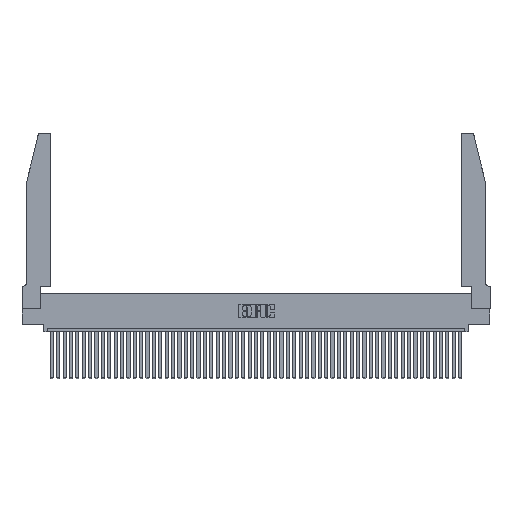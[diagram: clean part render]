
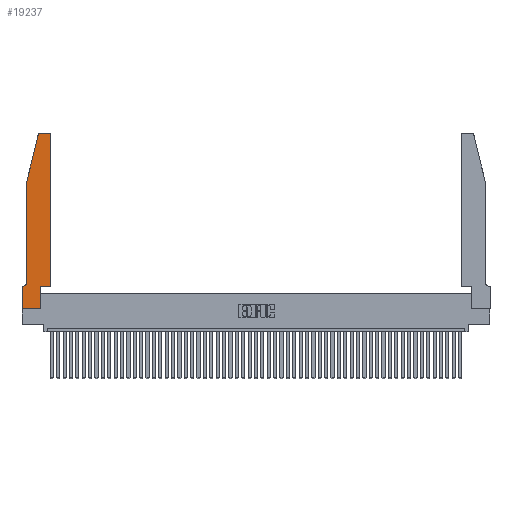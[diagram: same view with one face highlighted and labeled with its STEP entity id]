
A CAD part, top view. The second image highlights one B-rep face of the part: STEP entity #19237.
In plain terms, the highlighted planar face has unit normal (0, 0, 1).
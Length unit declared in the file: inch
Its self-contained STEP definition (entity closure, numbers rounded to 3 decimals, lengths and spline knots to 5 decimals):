
#61 = EDGE_CURVE ( 'NONE', #42414, #43759, #48741, .T. ) ;
#209 = ORIENTED_EDGE ( 'NONE', *, *, #61, .T. ) ;
#306 = CARTESIAN_POINT ( 'NONE',  ( 0.2865, 0.35, 0.37 ) ) ;
#961 = VERTEX_POINT ( 'NONE', #9647 ) ;
#1024 = VECTOR ( 'NONE', #28221, 39.37008 ) ;
#1819 = AXIS2_PLACEMENT_3D ( 'NONE', #43867, #20244, #3870 ) ;
#2735 = VERTEX_POINT ( 'NONE', #21769 ) ;
#3261 = EDGE_CURVE ( 'NONE', #11601, #9640, #23402, .T. ) ;
#3870 = DIRECTION ( 'NONE',  ( 1., 0., 0. ) ) ;
#4337 = ORIENTED_EDGE ( 'NONE', *, *, #50461, .T. ) ;
#4387 = DIRECTION ( 'NONE',  ( 1., 0., 0. ) ) ;
#4841 = ORIENTED_EDGE ( 'NONE', *, *, #11356, .T. ) ;
#5420 = CARTESIAN_POINT ( 'NONE',  ( 0., 0., 0.37 ) ) ;
#6988 = CARTESIAN_POINT ( 'NONE',  ( 0.0755, 2., 0.37 ) ) ;
#8207 = VECTOR ( 'NONE', #48902, 39.37008 ) ;
#8547 = DIRECTION ( 'NONE',  ( 1., 0., 0. ) ) ;
#8623 = CARTESIAN_POINT ( 'NONE',  ( 0.4205, 2.72, 0.37 ) ) ;
#8668 = ORIENTED_EDGE ( 'NONE', *, *, #19113, .T. ) ;
#8963 = CARTESIAN_POINT ( 'NONE',  ( 0.4505, 0.35, 0.37 ) ) ;
#9640 = VERTEX_POINT ( 'NONE', #14006 ) ;
#9647 = CARTESIAN_POINT ( 'NONE',  ( 0.0755, 2., 0.37 ) ) ;
#9802 = CARTESIAN_POINT ( 'NONE',  ( 0.4505, 0.35, 0.37 ) ) ;
#10198 = CARTESIAN_POINT ( 'NONE',  ( 0.4505, 0.35, 0.37 ) ) ;
#10938 = DIRECTION ( 'NONE',  ( -1., 0., 0. ) ) ;
#11356 = EDGE_CURVE ( 'NONE', #43759, #25865, #27672, .T. ) ;
#11601 = VERTEX_POINT ( 'NONE', #49882 ) ;
#11651 = VECTOR ( 'NONE', #23410, 39.37008 ) ;
#11686 = ORIENTED_EDGE ( 'NONE', *, *, #27457, .T. ) ;
#14006 = CARTESIAN_POINT ( 'NONE',  ( 0.2865, 0.35, 0.37 ) ) ;
#14422 = LINE ( 'NONE', #35608, #1024 ) ;
#15511 = LINE ( 'NONE', #6988, #30215 ) ;
#16026 = ORIENTED_EDGE ( 'NONE', *, *, #16996, .T. ) ;
#16112 = LINE ( 'NONE', #37106, #28999 ) ;
#16417 = FACE_OUTER_BOUND ( 'NONE', #31442, .T. ) ;
#16522 = DIRECTION ( 'NONE',  ( 0., 1., 0. ) ) ;
#16827 = VERTEX_POINT ( 'NONE', #32578 ) ;
#16996 = EDGE_CURVE ( 'NONE', #9640, #42414, #46573, .T. ) ;
#17390 = ORIENTED_EDGE ( 'NONE', *, *, #43235, .T. ) ;
#17571 = DIRECTION ( 'NONE',  ( -1., 0., 0. ) ) ;
#18559 = CARTESIAN_POINT ( 'NONE',  ( 0.0055, 0.42, 0.37 ) ) ;
#19056 = DIRECTION ( 'NONE',  ( 0., 0., -1. ) ) ;
#19113 = EDGE_CURVE ( 'NONE', #2735, #23541, #37305, .T. ) ;
#19237 = ADVANCED_FACE ( 'NONE', ( #16417 ), #24416, .T. ) ;
#20008 = DIRECTION ( 'NONE',  ( 0., 0., 1. ) ) ;
#20244 = DIRECTION ( 'NONE',  ( 0., 0., 1. ) ) ;
#20583 = VECTOR ( 'NONE', #40377, 39.37008 ) ;
#21147 = CIRCLE ( 'NONE', #35214, 0.03 ) ;
#21298 = ORIENTED_EDGE ( 'NONE', *, *, #48529, .T. ) ;
#21769 = CARTESIAN_POINT ( 'NONE',  ( 0.0755, 0.42, 0.37 ) ) ;
#23210 = LINE ( 'NONE', #29241, #29387 ) ;
#23402 = LINE ( 'NONE', #306, #32045 ) ;
#23410 = DIRECTION ( 'NONE',  ( 0., -1., 0. ) ) ;
#23541 = VERTEX_POINT ( 'NONE', #44327 ) ;
#24019 = CARTESIAN_POINT ( 'NONE',  ( 0.4205, 2.75, 0.37 ) ) ;
#24234 = EDGE_CURVE ( 'NONE', #961, #2735, #41565, .T. ) ;
#24416 = PLANE ( 'NONE',  #1819 ) ;
#25865 = VERTEX_POINT ( 'NONE', #24019 ) ;
#25982 = CARTESIAN_POINT ( 'NONE',  ( 0.4505, 2.72, 0.37 ) ) ;
#26034 = ORIENTED_EDGE ( 'NONE', *, *, #3261, .T. ) ;
#27457 = EDGE_CURVE ( 'NONE', #25865, #49422, #16112, .T. ) ;
#27672 = CIRCLE ( 'NONE', #49746, 0.03 ) ;
#28221 = DIRECTION ( 'NONE',  ( 0., -1., 0. ) ) ;
#28999 = VECTOR ( 'NONE', #17571, 39.37008 ) ;
#29241 = CARTESIAN_POINT ( 'NONE',  ( 0.0755, 0.35, 0.37 ) ) ;
#29387 = VECTOR ( 'NONE', #45430, 39.37008 ) ;
#30215 = VECTOR ( 'NONE', #49750, 39.37008 ) ;
#31442 = EDGE_LOOP ( 'NONE', ( #11686, #36193, #17390, #33651, #8668, #21298, #48675, #4337, #26034, #16026, #209, #4841 ) ) ;
#32045 = VECTOR ( 'NONE', #16522, 39.37008 ) ;
#32578 = CARTESIAN_POINT ( 'NONE',  ( 0.25487, 2.72718, 0.37 ) ) ;
#33249 = EDGE_CURVE ( 'NONE', #49422, #16827, #21147, .T. ) ;
#33328 = CARTESIAN_POINT ( 'NONE',  ( 0., 0.35, 0.37 ) ) ;
#33651 = ORIENTED_EDGE ( 'NONE', *, *, #24234, .T. ) ;
#35214 = AXIS2_PLACEMENT_3D ( 'NONE', #43473, #20008, #8547 ) ;
#35608 = CARTESIAN_POINT ( 'NONE',  ( 0., 0., 0.37 ) ) ;
#36193 = ORIENTED_EDGE ( 'NONE', *, *, #33249, .T. ) ;
#37106 = CARTESIAN_POINT ( 'NONE',  ( 0.2605, 2.75, 0.37 ) ) ;
#37305 = CIRCLE ( 'NONE', #43903, 0.07 ) ;
#37480 = CARTESIAN_POINT ( 'NONE',  ( 0., 0., 0.37 ) ) ;
#38733 = VERTEX_POINT ( 'NONE', #33328 ) ;
#40377 = DIRECTION ( 'NONE',  ( 1., 0., 0. ) ) ;
#41025 = DIRECTION ( 'NONE',  ( 0., 1., 0. ) ) ;
#41565 = LINE ( 'NONE', #46801, #11651 ) ;
#42001 = CARTESIAN_POINT ( 'NONE',  ( 0.284, 2.75, 0.37 ) ) ;
#42089 = LINE ( 'NONE', #5420, #20583 ) ;
#42329 = EDGE_CURVE ( 'NONE', #38733, #43855, #14422, .T. ) ;
#42414 = VERTEX_POINT ( 'NONE', #8963 ) ;
#43235 = EDGE_CURVE ( 'NONE', #16827, #961, #15511, .T. ) ;
#43473 = CARTESIAN_POINT ( 'NONE',  ( 0.284, 2.72, 0.37 ) ) ;
#43759 = VERTEX_POINT ( 'NONE', #25982 ) ;
#43855 = VERTEX_POINT ( 'NONE', #37480 ) ;
#43867 = CARTESIAN_POINT ( 'NONE',  ( 0., 0.35, 0.37 ) ) ;
#43879 = DIRECTION ( 'NONE',  ( 0., 0., 1. ) ) ;
#43903 = AXIS2_PLACEMENT_3D ( 'NONE', #18559, #19056, #10938 ) ;
#44327 = CARTESIAN_POINT ( 'NONE',  ( 0.0055, 0.35, 0.37 ) ) ;
#45430 = DIRECTION ( 'NONE',  ( -1., 0., 0. ) ) ;
#46573 = LINE ( 'NONE', #10198, #8207 ) ;
#46801 = CARTESIAN_POINT ( 'NONE',  ( 0.0755, 2., 0.37 ) ) ;
#48529 = EDGE_CURVE ( 'NONE', #23541, #38733, #23210, .T. ) ;
#48675 = ORIENTED_EDGE ( 'NONE', *, *, #42329, .T. ) ;
#48741 = LINE ( 'NONE', #9802, #49974 ) ;
#48902 = DIRECTION ( 'NONE',  ( 1., 0., 0. ) ) ;
#49422 = VERTEX_POINT ( 'NONE', #42001 ) ;
#49746 = AXIS2_PLACEMENT_3D ( 'NONE', #8623, #43879, #4387 ) ;
#49750 = DIRECTION ( 'NONE',  ( -0.239, -0.971, 0. ) ) ;
#49882 = CARTESIAN_POINT ( 'NONE',  ( 0.2865, 0., 0.37 ) ) ;
#49974 = VECTOR ( 'NONE', #41025, 39.37008 ) ;
#50461 = EDGE_CURVE ( 'NONE', #43855, #11601, #42089, .T. ) ;
